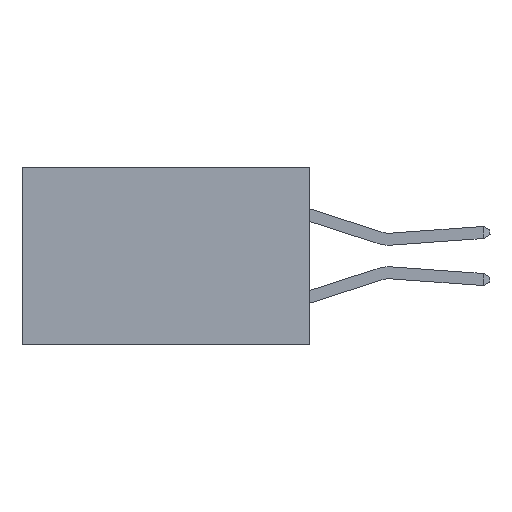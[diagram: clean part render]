
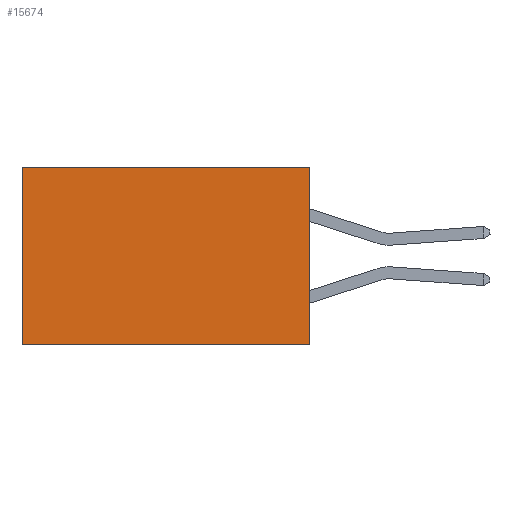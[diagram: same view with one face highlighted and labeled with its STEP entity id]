
A CAD part, left-side view. The second image highlights one B-rep face of the part: STEP entity #15674.
In plain terms, the highlighted planar face has unit normal (-1, 0, 0).
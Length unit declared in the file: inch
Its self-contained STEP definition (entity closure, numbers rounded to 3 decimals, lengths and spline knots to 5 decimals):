
#18 = FACE_OUTER_BOUND ( 'NONE', #4674, .T. ) ;
#735 = CARTESIAN_POINT ( 'NONE',  ( 0.2615, 0.6, -0.37 ) ) ;
#1295 = PLANE ( 'NONE',  #6412 ) ;
#1756 = LINE ( 'NONE', #735, #12951 ) ;
#2028 = CARTESIAN_POINT ( 'NONE',  ( 0.2615, 0.6, 0. ) ) ;
#2848 = CARTESIAN_POINT ( 'NONE',  ( 0.2615, 0., -0.37 ) ) ;
#2935 = CARTESIAN_POINT ( 'NONE',  ( 0.2615, 0.6, -0.37 ) ) ;
#3570 = ORIENTED_EDGE ( 'NONE', *, *, #17834, .T. ) ;
#3715 = ORIENTED_EDGE ( 'NONE', *, *, #15181, .F. ) ;
#3873 = VERTEX_POINT ( 'NONE', #17009 ) ;
#3962 = CARTESIAN_POINT ( 'NONE',  ( 0.2615, 0., 0. ) ) ;
#4182 = LINE ( 'NONE', #18047, #11488 ) ;
#4674 = EDGE_LOOP ( 'NONE', ( #3570, #3715, #8393, #13412 ) ) ;
#5697 = DIRECTION ( 'NONE',  ( 0., 1., 0. ) ) ;
#6313 = DIRECTION ( 'NONE',  ( 0., 0., -1. ) ) ;
#6412 = AXIS2_PLACEMENT_3D ( 'NONE', #2848, #11218, #6880 ) ;
#6601 = VERTEX_POINT ( 'NONE', #16005 ) ;
#6880 = DIRECTION ( 'NONE',  ( 0., 0., -1. ) ) ;
#7142 = EDGE_CURVE ( 'NONE', #3873, #6601, #7780, .T. ) ;
#7590 = VECTOR ( 'NONE', #5697, 39.37008 ) ;
#7780 = LINE ( 'NONE', #10657, #15147 ) ;
#8393 = ORIENTED_EDGE ( 'NONE', *, *, #7142, .F. ) ;
#10657 = CARTESIAN_POINT ( 'NONE',  ( 0.2615, 0., -0.37 ) ) ;
#10857 = EDGE_CURVE ( 'NONE', #3873, #12681, #12595, .T. ) ;
#10986 = DIRECTION ( 'NONE',  ( 0., 1., 0. ) ) ;
#11218 = DIRECTION ( 'NONE',  ( 1., 0., 0. ) ) ;
#11488 = VECTOR ( 'NONE', #10986, 39.37008 ) ;
#12595 = LINE ( 'NONE', #3962, #7590 ) ;
#12681 = VERTEX_POINT ( 'NONE', #2028 ) ;
#12951 = VECTOR ( 'NONE', #6313, 39.37008 ) ;
#13412 = ORIENTED_EDGE ( 'NONE', *, *, #10857, .T. ) ;
#14228 = VERTEX_POINT ( 'NONE', #2935 ) ;
#14597 = DIRECTION ( 'NONE',  ( 0., 0., -1. ) ) ;
#15147 = VECTOR ( 'NONE', #14597, 39.37008 ) ;
#15181 = EDGE_CURVE ( 'NONE', #6601, #14228, #4182, .T. ) ;
#15674 = ADVANCED_FACE ( 'NONE', ( #18 ), #1295, .F. ) ;
#16005 = CARTESIAN_POINT ( 'NONE',  ( 0.2615, 0., -0.37 ) ) ;
#17009 = CARTESIAN_POINT ( 'NONE',  ( 0.2615, 0., 0. ) ) ;
#17834 = EDGE_CURVE ( 'NONE', #12681, #14228, #1756, .T. ) ;
#18047 = CARTESIAN_POINT ( 'NONE',  ( 0.2615, 0., -0.37 ) ) ;
